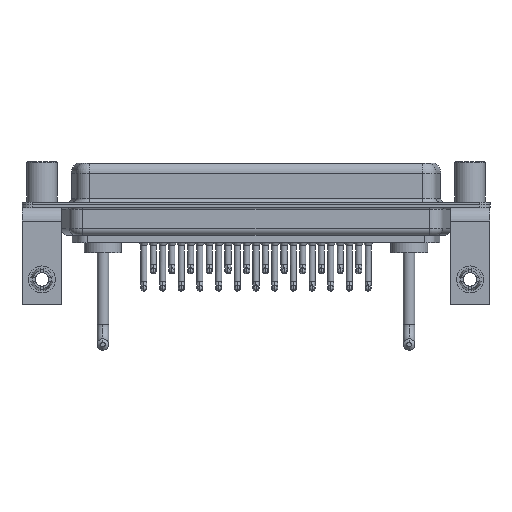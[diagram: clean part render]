
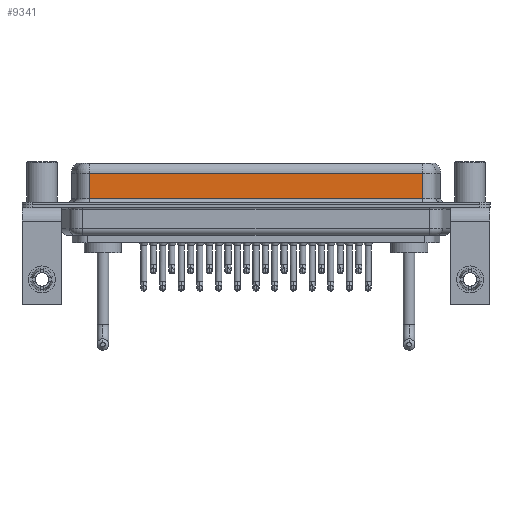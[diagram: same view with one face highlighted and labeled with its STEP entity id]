
A CAD part, front view. The second image highlights one B-rep face of the part: STEP entity #9341.
In plain terms, the highlighted planar face has unit normal (0, -1, 0).
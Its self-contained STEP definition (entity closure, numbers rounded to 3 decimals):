
#485 = CARTESIAN_POINT ( 'NONE',  ( 7.038, -3.95, 4.65 ) ) ;
#962 = ORIENTED_EDGE ( 'NONE', *, *, #13949, .F. ) ;
#4929 = EDGE_CURVE ( 'NONE', #8895, #8223, #23438, .T. ) ;
#5295 = CARTESIAN_POINT ( 'NONE',  ( 56.462, -3.95, 4.65 ) ) ;
#6151 = DIRECTION ( 'NONE',  ( 0., 1., 0. ) ) ;
#7965 = LINE ( 'NONE', #23785, #10286 ) ;
#8223 = VERTEX_POINT ( 'NONE', #25614 ) ;
#8483 = PLANE ( 'NONE',  #27729 ) ;
#8895 = VERTEX_POINT ( 'NONE', #28056 ) ;
#9341 = ADVANCED_FACE ( 'NONE', ( #28421 ), #8483, .F. ) ;
#10271 = VERTEX_POINT ( 'NONE', #485 ) ;
#10286 = VECTOR ( 'NONE', #23639, 1000. ) ;
#10949 = ORIENTED_EDGE ( 'NONE', *, *, #21006, .T. ) ;
#12029 = DIRECTION ( 'NONE',  ( -1., 0., 0. ) ) ;
#13536 = CARTESIAN_POINT ( 'NONE',  ( 56.462, -3.95, 6.4 ) ) ;
#13770 = ORIENTED_EDGE ( 'NONE', *, *, #4929, .T. ) ;
#13949 = EDGE_CURVE ( 'NONE', #21530, #8223, #27004, .T. ) ;
#14219 = DIRECTION ( 'NONE',  ( 1., 0., 0. ) ) ;
#16158 = DIRECTION ( 'NONE',  ( 0., 0., -1. ) ) ;
#16919 = ORIENTED_EDGE ( 'NONE', *, *, #17225, .T. ) ;
#17225 = EDGE_CURVE ( 'NONE', #21530, #10271, #25076, .T. ) ;
#17742 = CARTESIAN_POINT ( 'NONE',  ( 56.462, -3.95, 4.65 ) ) ;
#18271 = EDGE_LOOP ( 'NONE', ( #962, #16919, #10949, #13770 ) ) ;
#20486 = VECTOR ( 'NONE', #12029, 1000. ) ;
#21006 = EDGE_CURVE ( 'NONE', #10271, #8895, #7965, .T. ) ;
#21530 = VERTEX_POINT ( 'NONE', #17742 ) ;
#23438 = LINE ( 'NONE', #23582, #28522 ) ;
#23582 = CARTESIAN_POINT ( 'NONE',  ( 56.462, -3.95, 0.9 ) ) ;
#23639 = DIRECTION ( 'NONE',  ( 0., 0., -1. ) ) ;
#23785 = CARTESIAN_POINT ( 'NONE',  ( 7.038, -3.95, 6.4 ) ) ;
#24150 = VECTOR ( 'NONE', #16158, 1000. ) ;
#24311 = DIRECTION ( 'NONE',  ( 0., 0., 1. ) ) ;
#25076 = LINE ( 'NONE', #5295, #20486 ) ;
#25614 = CARTESIAN_POINT ( 'NONE',  ( 56.462, -3.95, 0.9 ) ) ;
#27004 = LINE ( 'NONE', #13536, #24150 ) ;
#27729 = AXIS2_PLACEMENT_3D ( 'NONE', #28127, #6151, #24311 ) ;
#28056 = CARTESIAN_POINT ( 'NONE',  ( 7.038, -3.95, 0.9 ) ) ;
#28127 = CARTESIAN_POINT ( 'NONE',  ( 56.462, -3.95, 6.4 ) ) ;
#28421 = FACE_OUTER_BOUND ( 'NONE', #18271, .T. ) ;
#28522 = VECTOR ( 'NONE', #14219, 1000. ) ;
